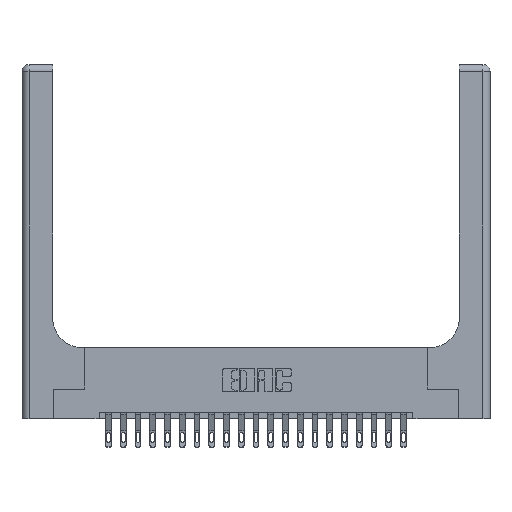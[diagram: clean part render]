
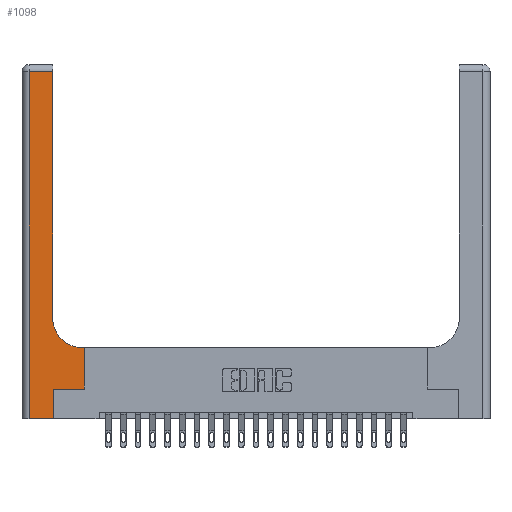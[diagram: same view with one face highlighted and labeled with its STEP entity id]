
A CAD part, top view. The second image highlights one B-rep face of the part: STEP entity #1098.
In plain terms, the highlighted planar face has unit normal (0, 0, 1).
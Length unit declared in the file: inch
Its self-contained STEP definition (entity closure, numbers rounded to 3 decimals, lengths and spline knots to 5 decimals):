
#85 = VECTOR ( 'NONE', #7276, 39.37008 ) ;
#371 = VERTEX_POINT ( 'NONE', #5874 ) ;
#526 = ORIENTED_EDGE ( 'NONE', *, *, #20526, .T. ) ;
#973 = AXIS2_PLACEMENT_3D ( 'NONE', #12445, #18666, #14725 ) ;
#1098 = ADVANCED_FACE ( 'NONE', ( #3322 ), #16128, .F. ) ;
#1221 = CARTESIAN_POINT ( 'NONE',  ( 0.26, 2.94, 0.37 ) ) ;
#1400 = VERTEX_POINT ( 'NONE', #5961 ) ;
#1624 = EDGE_CURVE ( 'NONE', #13739, #1400, #8051, .T. ) ;
#1634 = VERTEX_POINT ( 'NONE', #9731 ) ;
#1804 = VECTOR ( 'NONE', #4390, 39.37008 ) ;
#1970 = CARTESIAN_POINT ( 'NONE',  ( 0.06, 0., 0.37 ) ) ;
#2482 = ORIENTED_EDGE ( 'NONE', *, *, #4791, .T. ) ;
#2718 = EDGE_CURVE ( 'NONE', #1634, #20379, #7744, .T. ) ;
#3322 = FACE_OUTER_BOUND ( 'NONE', #19422, .T. ) ;
#3540 = ORIENTED_EDGE ( 'NONE', *, *, #17942, .T. ) ;
#3768 = CARTESIAN_POINT ( 'NONE',  ( 0.265, 0.25, 0.37 ) ) ;
#4118 = DIRECTION ( 'NONE',  ( 1., 0., 0. ) ) ;
#4273 = ORIENTED_EDGE ( 'NONE', *, *, #13862, .T. ) ;
#4390 = DIRECTION ( 'NONE',  ( 0., 1., 0. ) ) ;
#4515 = LINE ( 'NONE', #10872, #9317 ) ;
#4548 = ORIENTED_EDGE ( 'NONE', *, *, #2718, .T. ) ;
#4646 = VERTEX_POINT ( 'NONE', #3768 ) ;
#4748 = LINE ( 'NONE', #17519, #19698 ) ;
#4791 = EDGE_CURVE ( 'NONE', #371, #4646, #20430, .T. ) ;
#5874 = CARTESIAN_POINT ( 'NONE',  ( 0.265, 0., 0.37 ) ) ;
#5887 = VECTOR ( 'NONE', #18298, 39.37008 ) ;
#5961 = CARTESIAN_POINT ( 'NONE',  ( 0.26, 0.85, 0.37 ) ) ;
#6214 = EDGE_CURVE ( 'NONE', #20079, #13739, #19808, .T. ) ;
#6290 = ORIENTED_EDGE ( 'NONE', *, *, #1624, .T. ) ;
#6318 = LINE ( 'NONE', #12794, #1804 ) ;
#7276 = DIRECTION ( 'NONE',  ( -1., 0., 0. ) ) ;
#7744 = LINE ( 'NONE', #16588, #5887 ) ;
#7785 = EDGE_CURVE ( 'NONE', #17367, #1634, #13068, .T. ) ;
#8051 = CIRCLE ( 'NONE', #973, 0.25 ) ;
#8937 = CARTESIAN_POINT ( 'NONE',  ( 0.51, 0.6, 0.37 ) ) ;
#9001 = EDGE_CURVE ( 'NONE', #1400, #17367, #4748, .T. ) ;
#9317 = VECTOR ( 'NONE', #4118, 39.37008 ) ;
#9341 = VECTOR ( 'NONE', #19202, 39.37008 ) ;
#9699 = VERTEX_POINT ( 'NONE', #17574 ) ;
#9707 = ORIENTED_EDGE ( 'NONE', *, *, #9001, .T. ) ;
#9731 = CARTESIAN_POINT ( 'NONE',  ( 0.06, 2.94, 0.37 ) ) ;
#10872 = CARTESIAN_POINT ( 'NONE',  ( 0., 0., 0.37 ) ) ;
#11065 = CARTESIAN_POINT ( 'NONE',  ( 0.528, 0.6, 0.37 ) ) ;
#11611 = DIRECTION ( 'NONE',  ( 0., 1., 0. ) ) ;
#12445 = CARTESIAN_POINT ( 'NONE',  ( 0.51, 0.85, 0.37 ) ) ;
#12794 = CARTESIAN_POINT ( 'NONE',  ( 0.528, 0.25, 0.37 ) ) ;
#13068 = LINE ( 'NONE', #14077, #9341 ) ;
#13739 = VERTEX_POINT ( 'NONE', #8937 ) ;
#13862 = EDGE_CURVE ( 'NONE', #9699, #20079, #6318, .T. ) ;
#13873 = DIRECTION ( 'NONE',  ( 0., 1., 0. ) ) ;
#14077 = CARTESIAN_POINT ( 'NONE',  ( 0., 2.94, 0.37 ) ) ;
#14725 = DIRECTION ( 'NONE',  ( 1., 0., 0. ) ) ;
#14937 = ORIENTED_EDGE ( 'NONE', *, *, #6214, .T. ) ;
#15808 = AXIS2_PLACEMENT_3D ( 'NONE', #17825, #16261, #19405 ) ;
#15888 = VECTOR ( 'NONE', #11611, 39.37008 ) ;
#16128 = PLANE ( 'NONE',  #15808 ) ;
#16261 = DIRECTION ( 'NONE',  ( 0., 0., -1. ) ) ;
#16588 = CARTESIAN_POINT ( 'NONE',  ( 0.06, 3., 0.37 ) ) ;
#17367 = VERTEX_POINT ( 'NONE', #1221 ) ;
#17519 = CARTESIAN_POINT ( 'NONE',  ( 0.26, 3., 0.37 ) ) ;
#17574 = CARTESIAN_POINT ( 'NONE',  ( 0.528, 0.25, 0.37 ) ) ;
#17660 = CARTESIAN_POINT ( 'NONE',  ( 0.265, 0.25, 0.37 ) ) ;
#17825 = CARTESIAN_POINT ( 'NONE',  ( 0., 3., 0.37 ) ) ;
#17925 = LINE ( 'NONE', #17660, #20341 ) ;
#17942 = EDGE_CURVE ( 'NONE', #4646, #9699, #17925, .T. ) ;
#18191 = ORIENTED_EDGE ( 'NONE', *, *, #7785, .T. ) ;
#18298 = DIRECTION ( 'NONE',  ( 0., -1., 0. ) ) ;
#18666 = DIRECTION ( 'NONE',  ( 0., 0., -1. ) ) ;
#18894 = CARTESIAN_POINT ( 'NONE',  ( 0.26, 0.6, 0.37 ) ) ;
#19202 = DIRECTION ( 'NONE',  ( -1., 0., 0. ) ) ;
#19376 = DIRECTION ( 'NONE',  ( 1., 0., 0. ) ) ;
#19405 = DIRECTION ( 'NONE',  ( -1., 0., 0. ) ) ;
#19422 = EDGE_LOOP ( 'NONE', ( #9707, #18191, #4548, #526, #2482, #3540, #4273, #14937, #6290 ) ) ;
#19698 = VECTOR ( 'NONE', #13873, 39.37008 ) ;
#19808 = LINE ( 'NONE', #18894, #85 ) ;
#19894 = CARTESIAN_POINT ( 'NONE',  ( 0.265, 0., 0.37 ) ) ;
#20079 = VERTEX_POINT ( 'NONE', #11065 ) ;
#20341 = VECTOR ( 'NONE', #19376, 39.37008 ) ;
#20379 = VERTEX_POINT ( 'NONE', #1970 ) ;
#20430 = LINE ( 'NONE', #19894, #15888 ) ;
#20526 = EDGE_CURVE ( 'NONE', #20379, #371, #4515, .T. ) ;
